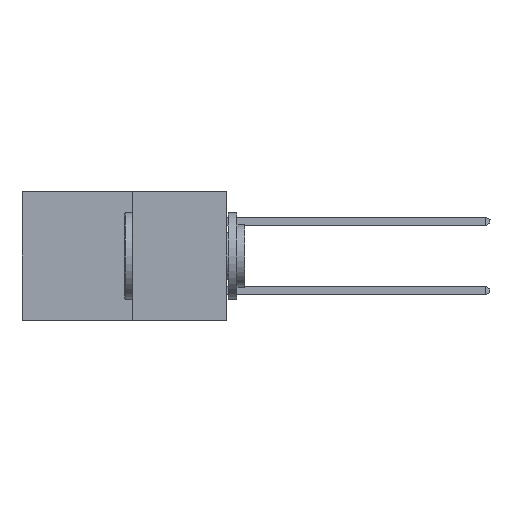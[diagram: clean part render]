
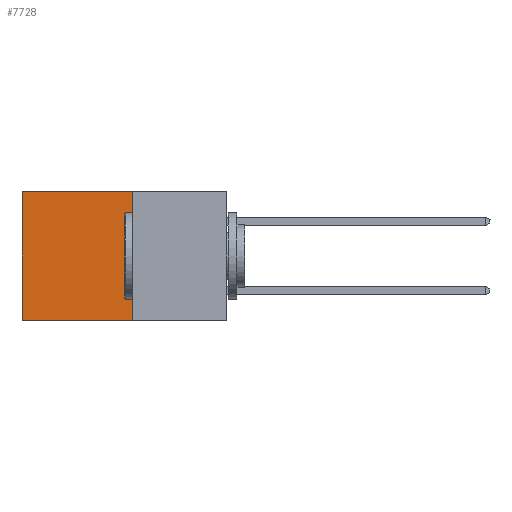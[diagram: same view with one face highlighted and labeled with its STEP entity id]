
A CAD part, left-side view. The second image highlights one B-rep face of the part: STEP entity #7728.
In plain terms, the highlighted planar face has unit normal (-1, 0, 0).
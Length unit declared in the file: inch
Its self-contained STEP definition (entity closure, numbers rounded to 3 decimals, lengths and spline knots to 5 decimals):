
#231 = VERTEX_POINT ( 'NONE', #7843 ) ;
#245 = EDGE_CURVE ( 'NONE', #853, #2130, #7717, .T. ) ;
#477 = VECTOR ( 'NONE', #6916, 39.37008 ) ;
#610 = DIRECTION ( 'NONE',  ( 0., 0., -1. ) ) ;
#853 = VERTEX_POINT ( 'NONE', #5528 ) ;
#1086 = CARTESIAN_POINT ( 'NONE',  ( 0.277, 0.27, -0.37 ) ) ;
#1204 = CARTESIAN_POINT ( 'NONE',  ( 0.277, 0.59, 0. ) ) ;
#1933 = EDGE_CURVE ( 'NONE', #231, #3714, #5332, .T. ) ;
#2049 = ORIENTED_EDGE ( 'NONE', *, *, #4706, .T. ) ;
#2130 = VERTEX_POINT ( 'NONE', #1204 ) ;
#3079 = LINE ( 'NONE', #7143, #477 ) ;
#3229 = FACE_OUTER_BOUND ( 'NONE', #4119, .T. ) ;
#3283 = VECTOR ( 'NONE', #5411, 39.37008 ) ;
#3469 = DIRECTION ( 'NONE',  ( 0., 1., 0. ) ) ;
#3609 = VECTOR ( 'NONE', #610, 39.37008 ) ;
#3707 = CARTESIAN_POINT ( 'NONE',  ( 0.277, 0.27, -0.37 ) ) ;
#3714 = VERTEX_POINT ( 'NONE', #9771 ) ;
#4119 = EDGE_LOOP ( 'NONE', ( #2049, #4335, #10615, #6806 ) ) ;
#4335 = ORIENTED_EDGE ( 'NONE', *, *, #1933, .F. ) ;
#4595 = DIRECTION ( 'NONE',  ( 0., 0., -1. ) ) ;
#4706 = EDGE_CURVE ( 'NONE', #2130, #3714, #3079, .T. ) ;
#5332 = LINE ( 'NONE', #3707, #7203 ) ;
#5411 = DIRECTION ( 'NONE',  ( 0., 1., 0. ) ) ;
#5528 = CARTESIAN_POINT ( 'NONE',  ( 0.277, 0.27, 0. ) ) ;
#6622 = CARTESIAN_POINT ( 'NONE',  ( 0.277, 0.27, -0.37 ) ) ;
#6806 = ORIENTED_EDGE ( 'NONE', *, *, #245, .T. ) ;
#6916 = DIRECTION ( 'NONE',  ( 0., 0., -1. ) ) ;
#7031 = PLANE ( 'NONE',  #10281 ) ;
#7143 = CARTESIAN_POINT ( 'NONE',  ( 0.277, 0.59, -0.37 ) ) ;
#7203 = VECTOR ( 'NONE', #3469, 39.37008 ) ;
#7717 = LINE ( 'NONE', #7875, #3283 ) ;
#7728 = ADVANCED_FACE ( 'NONE', ( #3229 ), #7031, .F. ) ;
#7843 = CARTESIAN_POINT ( 'NONE',  ( 0.277, 0.27, -0.37 ) ) ;
#7875 = CARTESIAN_POINT ( 'NONE',  ( 0.277, 0.27, 0. ) ) ;
#7990 = LINE ( 'NONE', #6622, #3609 ) ;
#9207 = EDGE_CURVE ( 'NONE', #853, #231, #7990, .T. ) ;
#9348 = DIRECTION ( 'NONE',  ( 1., 0., 0. ) ) ;
#9771 = CARTESIAN_POINT ( 'NONE',  ( 0.277, 0.59, -0.37 ) ) ;
#10281 = AXIS2_PLACEMENT_3D ( 'NONE', #1086, #9348, #4595 ) ;
#10615 = ORIENTED_EDGE ( 'NONE', *, *, #9207, .F. ) ;
